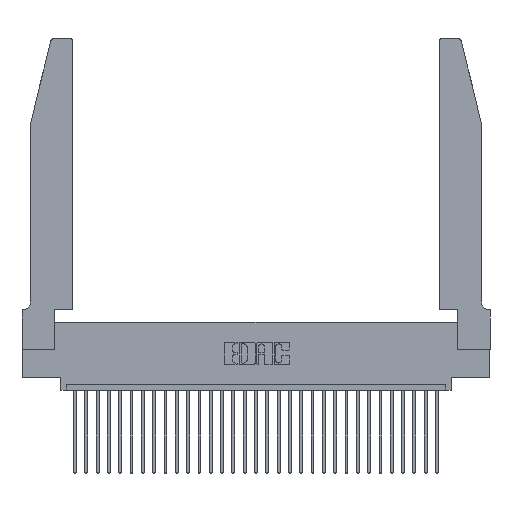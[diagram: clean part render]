
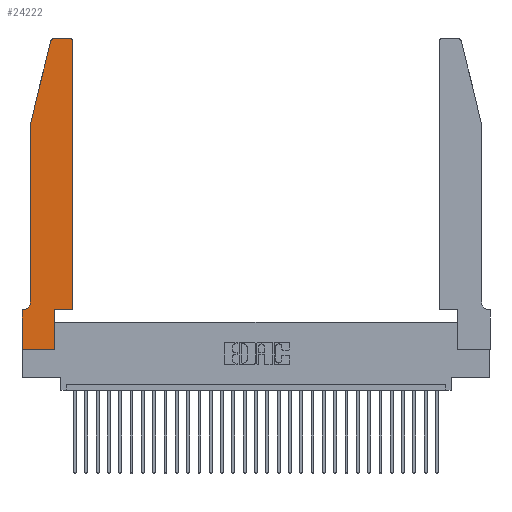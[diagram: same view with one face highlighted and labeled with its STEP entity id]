
A CAD part, top view. The second image highlights one B-rep face of the part: STEP entity #24222.
In plain terms, the highlighted planar face has unit normal (0, 0, 1).
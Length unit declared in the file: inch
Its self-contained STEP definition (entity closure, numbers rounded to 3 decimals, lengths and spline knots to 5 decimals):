
#537 = VERTEX_POINT ( 'NONE', #22911 ) ;
#1030 = CARTESIAN_POINT ( 'NONE',  ( 0.0755, 2., 0.37 ) ) ;
#1260 = DIRECTION ( 'NONE',  ( 1., 0., 0. ) ) ;
#1341 = DIRECTION ( 'NONE',  ( -1., 0., 0. ) ) ;
#1480 = DIRECTION ( 'NONE',  ( 0., -1., 0. ) ) ;
#1499 = EDGE_CURVE ( 'NONE', #26771, #537, #15410, .T. ) ;
#1952 = DIRECTION ( 'NONE',  ( 0., 0., 1. ) ) ;
#2031 = ORIENTED_EDGE ( 'NONE', *, *, #1499, .T. ) ;
#2096 = ORIENTED_EDGE ( 'NONE', *, *, #10952, .T. ) ;
#2272 = CARTESIAN_POINT ( 'NONE',  ( 0.0755, 2., 0.37 ) ) ;
#2727 = EDGE_CURVE ( 'NONE', #18641, #26771, #26210, .T. ) ;
#3712 = VERTEX_POINT ( 'NONE', #11854 ) ;
#3762 = ORIENTED_EDGE ( 'NONE', *, *, #10075, .T. ) ;
#3944 = EDGE_CURVE ( 'NONE', #19641, #29056, #28396, .T. ) ;
#4273 = DIRECTION ( 'NONE',  ( 1., 0., 0. ) ) ;
#4349 = VERTEX_POINT ( 'NONE', #2272 ) ;
#5056 = ORIENTED_EDGE ( 'NONE', *, *, #20696, .T. ) ;
#5216 = EDGE_CURVE ( 'NONE', #22150, #21809, #25618, .T. ) ;
#6631 = CARTESIAN_POINT ( 'NONE',  ( 0.0055, 0.42, 0.37 ) ) ;
#6832 = LINE ( 'NONE', #29629, #11631 ) ;
#7320 = CARTESIAN_POINT ( 'NONE',  ( 0.0755, 0.42, 0.37 ) ) ;
#7448 = EDGE_CURVE ( 'NONE', #11248, #3712, #18326, .T. ) ;
#8331 = FACE_OUTER_BOUND ( 'NONE', #26554, .T. ) ;
#8542 = EDGE_CURVE ( 'NONE', #21809, #4349, #29877, .T. ) ;
#8625 = CARTESIAN_POINT ( 'NONE',  ( 0.284, 2.75, 0.37 ) ) ;
#8686 = CARTESIAN_POINT ( 'NONE',  ( 0., 0.35, 0.37 ) ) ;
#8765 = CARTESIAN_POINT ( 'NONE',  ( 0.0755, 0.35, 0.37 ) ) ;
#9084 = DIRECTION ( 'NONE',  ( 1., 0., 0. ) ) ;
#9418 = CARTESIAN_POINT ( 'NONE',  ( 0.2865, 0.35, 0.37 ) ) ;
#9663 = CARTESIAN_POINT ( 'NONE',  ( 0.4205, 2.75, 0.37 ) ) ;
#9674 = CARTESIAN_POINT ( 'NONE',  ( 0.4205, 2.72, 0.37 ) ) ;
#9916 = LINE ( 'NONE', #25255, #26397 ) ;
#10075 = EDGE_CURVE ( 'NONE', #3712, #13195, #11037, .T. ) ;
#10714 = EDGE_CURVE ( 'NONE', #537, #14030, #23390, .T. ) ;
#10952 = EDGE_CURVE ( 'NONE', #29056, #22150, #9916, .T. ) ;
#11037 = LINE ( 'NONE', #8765, #15922 ) ;
#11129 = AXIS2_PLACEMENT_3D ( 'NONE', #28199, #1952, #4273 ) ;
#11248 = VERTEX_POINT ( 'NONE', #7320 ) ;
#11484 = DIRECTION ( 'NONE',  ( 0., 0., -1. ) ) ;
#11631 = VECTOR ( 'NONE', #22487, 39.37008 ) ;
#11641 = AXIS2_PLACEMENT_3D ( 'NONE', #28931, #26212, #14587 ) ;
#11854 = CARTESIAN_POINT ( 'NONE',  ( 0.0055, 0.35, 0.37 ) ) ;
#12026 = CARTESIAN_POINT ( 'NONE',  ( 0.4505, 2.72, 0.37 ) ) ;
#13195 = VERTEX_POINT ( 'NONE', #8686 ) ;
#13262 = EDGE_CURVE ( 'NONE', #13195, #18641, #23270, .T. ) ;
#13531 = VECTOR ( 'NONE', #14313, 39.37008 ) ;
#13566 = CARTESIAN_POINT ( 'NONE',  ( 0., 0., 0.37 ) ) ;
#14030 = VERTEX_POINT ( 'NONE', #25208 ) ;
#14313 = DIRECTION ( 'NONE',  ( 0., 1., 0. ) ) ;
#14587 = DIRECTION ( 'NONE',  ( 1., 0., 0. ) ) ;
#14618 = EDGE_CURVE ( 'NONE', #14030, #19641, #19045, .T. ) ;
#15410 = LINE ( 'NONE', #9418, #13531 ) ;
#15451 = CARTESIAN_POINT ( 'NONE',  ( 0.2865, 0., 0.37 ) ) ;
#15627 = CARTESIAN_POINT ( 'NONE',  ( 0.4505, 0.35, 0.37 ) ) ;
#15922 = VECTOR ( 'NONE', #18447, 39.37008 ) ;
#16469 = ORIENTED_EDGE ( 'NONE', *, *, #7448, .T. ) ;
#16471 = DIRECTION ( 'NONE',  ( 0., 0., 1. ) ) ;
#17214 = VECTOR ( 'NONE', #9084, 39.37008 ) ;
#18326 = CIRCLE ( 'NONE', #29958, 0.07 ) ;
#18447 = DIRECTION ( 'NONE',  ( -1., 0., 0. ) ) ;
#18641 = VERTEX_POINT ( 'NONE', #13566 ) ;
#18795 = CARTESIAN_POINT ( 'NONE',  ( 0.25487, 2.72718, 0.37 ) ) ;
#19045 = LINE ( 'NONE', #15627, #26555 ) ;
#19118 = ORIENTED_EDGE ( 'NONE', *, *, #3944, .T. ) ;
#19641 = VERTEX_POINT ( 'NONE', #12026 ) ;
#20231 = DIRECTION ( 'NONE',  ( -0.239, -0.971, 0. ) ) ;
#20696 = EDGE_CURVE ( 'NONE', #4349, #11248, #6832, .T. ) ;
#20982 = ORIENTED_EDGE ( 'NONE', *, *, #8542, .T. ) ;
#21161 = PLANE ( 'NONE',  #11129 ) ;
#21661 = ORIENTED_EDGE ( 'NONE', *, *, #14618, .T. ) ;
#21809 = VERTEX_POINT ( 'NONE', #18795 ) ;
#22150 = VERTEX_POINT ( 'NONE', #8625 ) ;
#22262 = ORIENTED_EDGE ( 'NONE', *, *, #2727, .T. ) ;
#22475 = AXIS2_PLACEMENT_3D ( 'NONE', #9674, #16471, #30671 ) ;
#22487 = DIRECTION ( 'NONE',  ( 0., -1., 0. ) ) ;
#22911 = CARTESIAN_POINT ( 'NONE',  ( 0.2865, 0.35, 0.37 ) ) ;
#23270 = LINE ( 'NONE', #30117, #27808 ) ;
#23390 = LINE ( 'NONE', #25076, #30483 ) ;
#24066 = DIRECTION ( 'NONE',  ( 0., 1., 0. ) ) ;
#24222 = ADVANCED_FACE ( 'NONE', ( #8331 ), #21161, .T. ) ;
#24754 = ORIENTED_EDGE ( 'NONE', *, *, #13262, .T. ) ;
#25076 = CARTESIAN_POINT ( 'NONE',  ( 0.4505, 0.35, 0.37 ) ) ;
#25208 = CARTESIAN_POINT ( 'NONE',  ( 0.4505, 0.35, 0.37 ) ) ;
#25255 = CARTESIAN_POINT ( 'NONE',  ( 0.2605, 2.75, 0.37 ) ) ;
#25618 = CIRCLE ( 'NONE', #11641, 0.03 ) ;
#25958 = ORIENTED_EDGE ( 'NONE', *, *, #5216, .T. ) ;
#26210 = LINE ( 'NONE', #30490, #17214 ) ;
#26212 = DIRECTION ( 'NONE',  ( 0., 0., 1. ) ) ;
#26397 = VECTOR ( 'NONE', #1341, 39.37008 ) ;
#26554 = EDGE_LOOP ( 'NONE', ( #2096, #25958, #20982, #5056, #16469, #3762, #24754, #22262, #2031, #29726, #21661, #19118 ) ) ;
#26555 = VECTOR ( 'NONE', #24066, 39.37008 ) ;
#26771 = VERTEX_POINT ( 'NONE', #15451 ) ;
#27646 = VECTOR ( 'NONE', #20231, 39.37008 ) ;
#27808 = VECTOR ( 'NONE', #1480, 39.37008 ) ;
#28199 = CARTESIAN_POINT ( 'NONE',  ( 0., 0.35, 0.37 ) ) ;
#28272 = DIRECTION ( 'NONE',  ( -1., 0., 0. ) ) ;
#28396 = CIRCLE ( 'NONE', #22475, 0.03 ) ;
#28931 = CARTESIAN_POINT ( 'NONE',  ( 0.284, 2.72, 0.37 ) ) ;
#29056 = VERTEX_POINT ( 'NONE', #9663 ) ;
#29629 = CARTESIAN_POINT ( 'NONE',  ( 0.0755, 2., 0.37 ) ) ;
#29726 = ORIENTED_EDGE ( 'NONE', *, *, #10714, .T. ) ;
#29877 = LINE ( 'NONE', #1030, #27646 ) ;
#29958 = AXIS2_PLACEMENT_3D ( 'NONE', #6631, #11484, #28272 ) ;
#30117 = CARTESIAN_POINT ( 'NONE',  ( 0., 0., 0.37 ) ) ;
#30483 = VECTOR ( 'NONE', #1260, 39.37008 ) ;
#30490 = CARTESIAN_POINT ( 'NONE',  ( 0., 0., 0.37 ) ) ;
#30671 = DIRECTION ( 'NONE',  ( 1., 0., 0. ) ) ;
